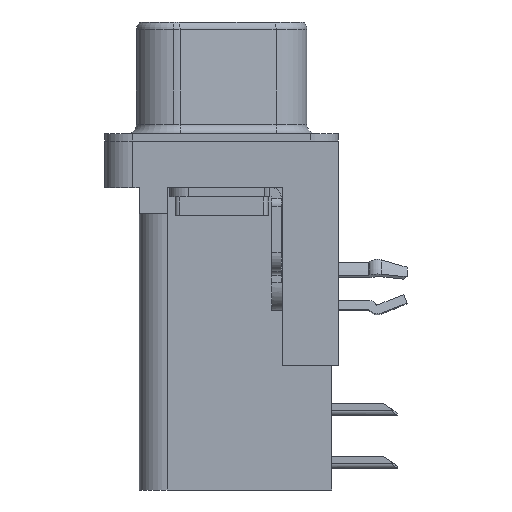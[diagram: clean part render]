
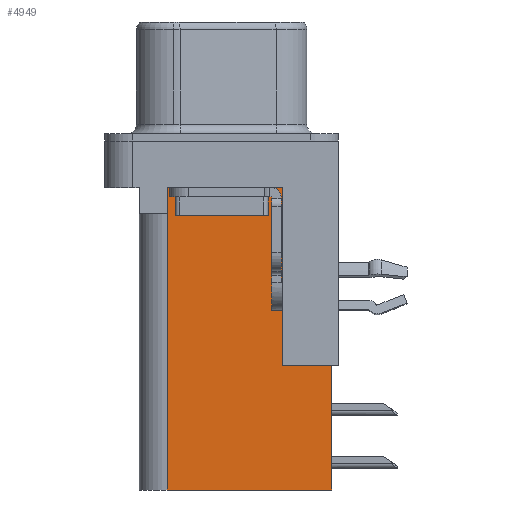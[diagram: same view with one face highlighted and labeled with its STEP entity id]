
A CAD part, left-side view. The second image highlights one B-rep face of the part: STEP entity #4949.
In plain terms, the highlighted planar face has unit normal (-1, 0, 0).
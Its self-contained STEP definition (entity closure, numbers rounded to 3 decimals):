
#327 = ORIENTED_EDGE ( 'NONE', *, *, #8047, .T. ) ;
#605 = DIRECTION ( 'NONE',  ( 0., 0., 1. ) ) ;
#1123 = CARTESIAN_POINT ( 'NONE',  ( 3.79, -5.925, -2. ) ) ;
#1266 = VECTOR ( 'NONE', #2674, 1000. ) ;
#1439 = VERTEX_POINT ( 'NONE', #10550 ) ;
#1596 = VECTOR ( 'NONE', #14421, 1000. ) ;
#1923 = EDGE_CURVE ( 'NONE', #12454, #6929, #11270, .T. ) ;
#2558 = CARTESIAN_POINT ( 'NONE',  ( 3.79, -5.925, -12.05 ) ) ;
#2674 = DIRECTION ( 'NONE',  ( 0., 1., 0. ) ) ;
#2838 = VERTEX_POINT ( 'NONE', #2558 ) ;
#3892 = VERTEX_POINT ( 'NONE', #11521 ) ;
#4007 = CARTESIAN_POINT ( 'NONE',  ( 3.79, 2.925, -18.76 ) ) ;
#4055 = ORIENTED_EDGE ( 'NONE', *, *, #8788, .T. ) ;
#4760 = CARTESIAN_POINT ( 'NONE',  ( 3.79, 0., -3.9 ) ) ;
#4767 = DIRECTION ( 'NONE',  ( 0., 0., -1. ) ) ;
#4839 = CARTESIAN_POINT ( 'NONE',  ( 3.79, -6.295, -12.05 ) ) ;
#4937 = ORIENTED_EDGE ( 'NONE', *, *, #15059, .F. ) ;
#4949 = ADVANCED_FACE ( 'NONE', ( #15030 ), #13751, .F. ) ;
#5486 = CARTESIAN_POINT ( 'NONE',  ( 3.79, -3.295, -18.76 ) ) ;
#5692 = VECTOR ( 'NONE', #4767, 1000. ) ;
#5694 = CARTESIAN_POINT ( 'NONE',  ( 3.79, -3.295, -2.5 ) ) ;
#5980 = VECTOR ( 'NONE', #8343, 1000. ) ;
#6171 = VECTOR ( 'NONE', #605, 1000. ) ;
#6726 = DIRECTION ( 'NONE',  ( 0., 1., 0. ) ) ;
#6929 = VERTEX_POINT ( 'NONE', #5694 ) ;
#7606 = DIRECTION ( 'NONE',  ( 0., 0., -1. ) ) ;
#7624 = VERTEX_POINT ( 'NONE', #4007 ) ;
#7700 = ORIENTED_EDGE ( 'NONE', *, *, #1923, .T. ) ;
#7815 = CARTESIAN_POINT ( 'NONE',  ( 3.79, 2.925, -18.76 ) ) ;
#8047 = EDGE_CURVE ( 'NONE', #13162, #3892, #8739, .T. ) ;
#8211 = CARTESIAN_POINT ( 'NONE',  ( 3.79, -5.925, -18.76 ) ) ;
#8343 = DIRECTION ( 'NONE',  ( 0., 1., 0. ) ) ;
#8373 = VECTOR ( 'NONE', #7606, 1000. ) ;
#8739 = LINE ( 'NONE', #15686, #8373 ) ;
#8788 = EDGE_CURVE ( 'NONE', #6929, #13162, #10935, .T. ) ;
#8904 = LINE ( 'NONE', #1123, #5692 ) ;
#9006 = AXIS2_PLACEMENT_3D ( 'NONE', #11761, #9234, #9034 ) ;
#9034 = DIRECTION ( 'NONE',  ( 0., 1., 0. ) ) ;
#9172 = EDGE_CURVE ( 'NONE', #3892, #1439, #12462, .T. ) ;
#9234 = DIRECTION ( 'NONE',  ( 1., 0., 0. ) ) ;
#9387 = LINE ( 'NONE', #7815, #6171 ) ;
#10253 = CARTESIAN_POINT ( 'NONE',  ( 3.79, -3.295, -12.05 ) ) ;
#10550 = CARTESIAN_POINT ( 'NONE',  ( 3.79, 2.925, -3.9 ) ) ;
#10685 = VERTEX_POINT ( 'NONE', #8211 ) ;
#10785 = ORIENTED_EDGE ( 'NONE', *, *, #14640, .F. ) ;
#10848 = VECTOR ( 'NONE', #6726, 1000. ) ;
#10935 = LINE ( 'NONE', #13565, #1266 ) ;
#11233 = LINE ( 'NONE', #5486, #10848 ) ;
#11270 = LINE ( 'NONE', #14202, #1596 ) ;
#11521 = CARTESIAN_POINT ( 'NONE',  ( 3.79, 2.895, -3.9 ) ) ;
#11761 = CARTESIAN_POINT ( 'NONE',  ( 3.79, -3.295, -18.76 ) ) ;
#11844 = EDGE_CURVE ( 'NONE', #7624, #1439, #9387, .T. ) ;
#11862 = ORIENTED_EDGE ( 'NONE', *, *, #9172, .T. ) ;
#12238 = VECTOR ( 'NONE', #13351, 1000. ) ;
#12454 = VERTEX_POINT ( 'NONE', #10253 ) ;
#12462 = LINE ( 'NONE', #4760, #5980 ) ;
#12781 = EDGE_CURVE ( 'NONE', #2838, #12454, #15168, .T. ) ;
#13124 = ORIENTED_EDGE ( 'NONE', *, *, #12781, .T. ) ;
#13162 = VERTEX_POINT ( 'NONE', #14176 ) ;
#13351 = DIRECTION ( 'NONE',  ( 0., 1., 0. ) ) ;
#13565 = CARTESIAN_POINT ( 'NONE',  ( 3.79, -3.295, -2.5 ) ) ;
#13751 = PLANE ( 'NONE',  #9006 ) ;
#13988 = EDGE_LOOP ( 'NONE', ( #4055, #327, #11862, #15409, #4937, #10785, #13124, #7700 ) ) ;
#14176 = CARTESIAN_POINT ( 'NONE',  ( 3.79, 2.895, -2.5 ) ) ;
#14202 = CARTESIAN_POINT ( 'NONE',  ( 3.79, -3.295, -18.76 ) ) ;
#14421 = DIRECTION ( 'NONE',  ( 0., 0., 1. ) ) ;
#14640 = EDGE_CURVE ( 'NONE', #2838, #10685, #8904, .T. ) ;
#15030 = FACE_OUTER_BOUND ( 'NONE', #13988, .T. ) ;
#15059 = EDGE_CURVE ( 'NONE', #10685, #7624, #11233, .T. ) ;
#15168 = LINE ( 'NONE', #4839, #12238 ) ;
#15409 = ORIENTED_EDGE ( 'NONE', *, *, #11844, .F. ) ;
#15686 = CARTESIAN_POINT ( 'NONE',  ( 3.79, 2.895, -3.9 ) ) ;
